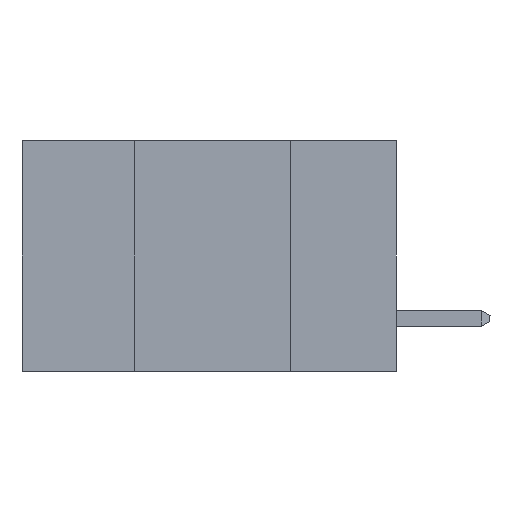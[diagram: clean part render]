
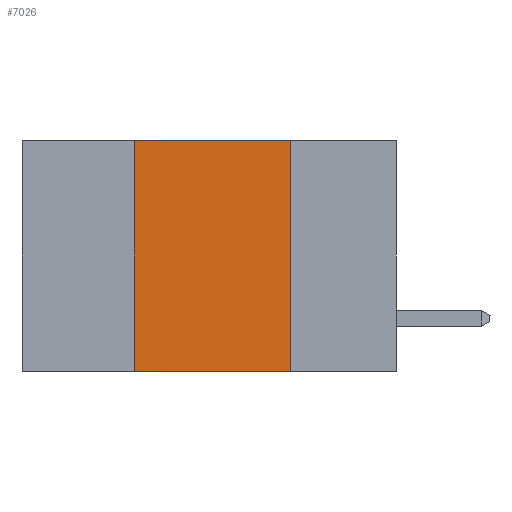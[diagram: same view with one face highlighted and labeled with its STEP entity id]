
A CAD part, left-side view. The second image highlights one B-rep face of the part: STEP entity #7026.
In plain terms, the highlighted planar face has unit normal (-1, 0, 0).
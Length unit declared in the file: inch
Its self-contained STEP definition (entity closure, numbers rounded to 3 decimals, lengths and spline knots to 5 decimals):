
#219 = VERTEX_POINT ( 'NONE', #5106 ) ;
#974 = LINE ( 'NONE', #4401, #7726 ) ;
#1095 = FACE_OUTER_BOUND ( 'NONE', #3174, .T. ) ;
#1443 = EDGE_CURVE ( 'NONE', #219, #2564, #5635, .T. ) ;
#1634 = DIRECTION ( 'NONE',  ( 0., 0., -1. ) ) ;
#1647 = VERTEX_POINT ( 'NONE', #5220 ) ;
#2077 = VERTEX_POINT ( 'NONE', #7594 ) ;
#2564 = VERTEX_POINT ( 'NONE', #2863 ) ;
#2713 = DIRECTION ( 'NONE',  ( 0., 0., 1. ) ) ;
#2863 = CARTESIAN_POINT ( 'NONE',  ( 0., 0.17, -0.37 ) ) ;
#3174 = EDGE_LOOP ( 'NONE', ( #7998, #5792, #9554, #5070 ) ) ;
#3483 = AXIS2_PLACEMENT_3D ( 'NONE', #9280, #6787, #10007 ) ;
#3587 = PLANE ( 'NONE',  #3483 ) ;
#4401 = CARTESIAN_POINT ( 'NONE',  ( 0., 0.42, -0.37 ) ) ;
#5016 = DIRECTION ( 'NONE',  ( 0., -1., 0. ) ) ;
#5070 = ORIENTED_EDGE ( 'NONE', *, *, #6859, .T. ) ;
#5106 = CARTESIAN_POINT ( 'NONE',  ( 0., 0.17, 0. ) ) ;
#5220 = CARTESIAN_POINT ( 'NONE',  ( 0., 0.42, 0. ) ) ;
#5279 = CARTESIAN_POINT ( 'NONE',  ( 0., 0.6, -0.37 ) ) ;
#5635 = LINE ( 'NONE', #8873, #9640 ) ;
#5792 = ORIENTED_EDGE ( 'NONE', *, *, #10210, .F. ) ;
#5814 = VECTOR ( 'NONE', #8565, 39.37008 ) ;
#5961 = CARTESIAN_POINT ( 'NONE',  ( 0., 0.6, 0. ) ) ;
#6120 = LINE ( 'NONE', #5279, #5814 ) ;
#6787 = DIRECTION ( 'NONE',  ( 1., 0., 0. ) ) ;
#6859 = EDGE_CURVE ( 'NONE', #2077, #2564, #6120, .T. ) ;
#7026 = ADVANCED_FACE ( 'NONE', ( #1095 ), #3587, .F. ) ;
#7570 = VECTOR ( 'NONE', #5016, 39.37008 ) ;
#7594 = CARTESIAN_POINT ( 'NONE',  ( 0., 0.42, -0.37 ) ) ;
#7726 = VECTOR ( 'NONE', #2713, 39.37008 ) ;
#7998 = ORIENTED_EDGE ( 'NONE', *, *, #1443, .F. ) ;
#8299 = LINE ( 'NONE', #5961, #7570 ) ;
#8565 = DIRECTION ( 'NONE',  ( 0., -1., 0. ) ) ;
#8873 = CARTESIAN_POINT ( 'NONE',  ( 0., 0.17, -0.37 ) ) ;
#9280 = CARTESIAN_POINT ( 'NONE',  ( 0., 0.6, 0. ) ) ;
#9554 = ORIENTED_EDGE ( 'NONE', *, *, #9834, .F. ) ;
#9640 = VECTOR ( 'NONE', #1634, 39.37008 ) ;
#9834 = EDGE_CURVE ( 'NONE', #2077, #1647, #974, .T. ) ;
#10007 = DIRECTION ( 'NONE',  ( 0., 0., -1. ) ) ;
#10210 = EDGE_CURVE ( 'NONE', #1647, #219, #8299, .T. ) ;
